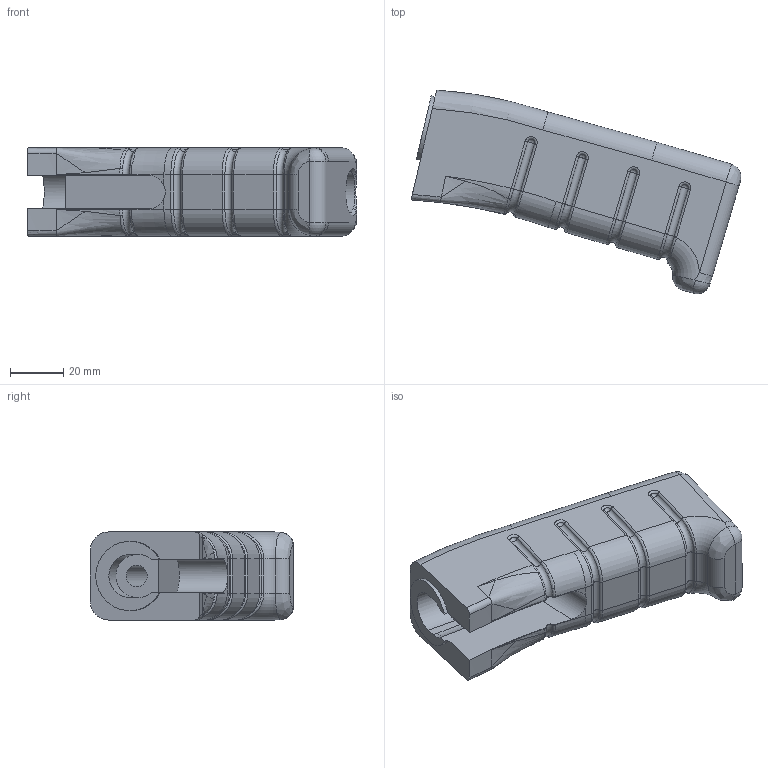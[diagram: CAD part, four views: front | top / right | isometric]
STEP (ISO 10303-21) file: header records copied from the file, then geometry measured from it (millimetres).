
FILE_DESCRIPTION(/* description */ (''),/* implementation_level */ '2;1');
FILE_NAME(/* name */ 'Hatfield Grip.step',/* time_stamp */ '2021-05-20T08:37:02-06:00',/* author */ (''),/* organization */ (''),/* preprocessor_version */ 'ST-DEVELOPER v18.1',/* originating_system */ 'Autodesk Translation Framework v10.6.0.1341',/* authorisation */ '');
FILE_SCHEMA (('AUTOMOTIVE_DESIGN { 1 0 10303 214 3 1 1 }'));
Length unit declared in the file: millimetre
Products named in the file (1): Hatfield Projects
Bounding box: 123.56 x 76.23 x 33 mm (x, y, z)
Volume: 134891.1 mm3; surface area: 25045.4 mm2
Topology: 1 solids, 1 shells, 281 faces, 727 edges, 446 vertices
Faces by surface type: plane 83, bspline 81, cylinder 69, torus 38, sphere 10
Full cylindrical faces by diameter (mm): 8 x1, 15.5 x1
Entity records: 11035 total; most frequent: CARTESIAN_POINT 4681, ORIENTED_EDGE 1436, DIRECTION 1197, EDGE_CURVE 718, AXIS2_PLACEMENT_3D 447, VERTEX_POINT 446, LINE 303, VECTOR 303
